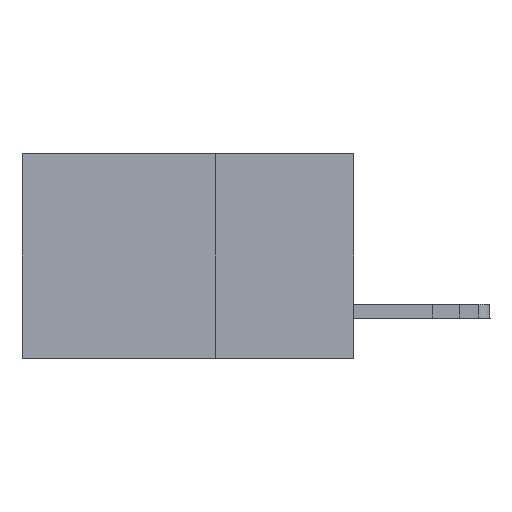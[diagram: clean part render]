
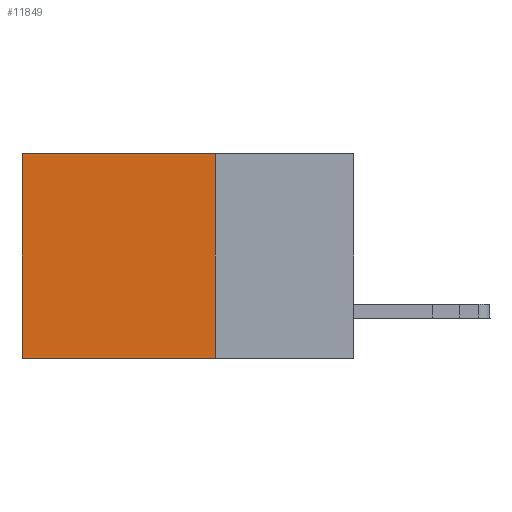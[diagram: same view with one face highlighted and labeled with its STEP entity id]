
A CAD part, left-side view. The second image highlights one B-rep face of the part: STEP entity #11849.
In plain terms, the highlighted planar face has unit normal (-1, 0, 0).
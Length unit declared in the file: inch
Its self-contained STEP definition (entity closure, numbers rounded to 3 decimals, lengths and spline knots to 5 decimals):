
#397 = DIRECTION ( 'NONE',  ( 0., 1., 0. ) ) ;
#1857 = CARTESIAN_POINT ( 'NONE',  ( 0.2875, 0.6, 0. ) ) ;
#2567 = VECTOR ( 'NONE', #23608, 39.37008 ) ;
#2897 = ORIENTED_EDGE ( 'NONE', *, *, #4030, .F. ) ;
#2952 = CARTESIAN_POINT ( 'NONE',  ( 0.2875, 0.25, 0. ) ) ;
#3026 = LINE ( 'NONE', #13489, #25670 ) ;
#3095 = ORIENTED_EDGE ( 'NONE', *, *, #11351, .T. ) ;
#3740 = VECTOR ( 'NONE', #397, 39.37008 ) ;
#4030 = EDGE_CURVE ( 'NONE', #10977, #20975, #3026, .T. ) ;
#5952 = VERTEX_POINT ( 'NONE', #2952 ) ;
#7763 = EDGE_CURVE ( 'NONE', #5952, #10977, #14908, .T. ) ;
#9144 = EDGE_CURVE ( 'NONE', #24712, #20975, #12087, .T. ) ;
#10121 = CARTESIAN_POINT ( 'NONE',  ( 0.2875, 0.25, -0.37 ) ) ;
#10652 = DIRECTION ( 'NONE',  ( 1., 0., 0. ) ) ;
#10977 = VERTEX_POINT ( 'NONE', #10121 ) ;
#11351 = EDGE_CURVE ( 'NONE', #5952, #24712, #21190, .T. ) ;
#11849 = ADVANCED_FACE ( 'NONE', ( #12816 ), #26188, .F. ) ;
#12087 = LINE ( 'NONE', #15108, #17179 ) ;
#12816 = FACE_OUTER_BOUND ( 'NONE', #22720, .T. ) ;
#13489 = CARTESIAN_POINT ( 'NONE',  ( 0.2875, 0.25, -0.37 ) ) ;
#14557 = ORIENTED_EDGE ( 'NONE', *, *, #7763, .F. ) ;
#14908 = LINE ( 'NONE', #21387, #2567 ) ;
#15108 = CARTESIAN_POINT ( 'NONE',  ( 0.2875, 0.6, 0. ) ) ;
#17179 = VECTOR ( 'NONE', #17284, 39.37008 ) ;
#17284 = DIRECTION ( 'NONE',  ( 0., 0., -1. ) ) ;
#17630 = ORIENTED_EDGE ( 'NONE', *, *, #9144, .T. ) ;
#20975 = VERTEX_POINT ( 'NONE', #26289 ) ;
#21190 = LINE ( 'NONE', #26684, #3740 ) ;
#21387 = CARTESIAN_POINT ( 'NONE',  ( 0.2875, 0.25, 0. ) ) ;
#22720 = EDGE_LOOP ( 'NONE', ( #17630, #2897, #14557, #3095 ) ) ;
#23608 = DIRECTION ( 'NONE',  ( 0., 0., -1. ) ) ;
#23948 = CARTESIAN_POINT ( 'NONE',  ( 0.2875, 0.25, 0. ) ) ;
#24712 = VERTEX_POINT ( 'NONE', #1857 ) ;
#25670 = VECTOR ( 'NONE', #26637, 39.37008 ) ;
#26188 = PLANE ( 'NONE',  #26867 ) ;
#26289 = CARTESIAN_POINT ( 'NONE',  ( 0.2875, 0.6, -0.37 ) ) ;
#26637 = DIRECTION ( 'NONE',  ( 0., 1., 0. ) ) ;
#26684 = CARTESIAN_POINT ( 'NONE',  ( 0.2875, 0.25, 0. ) ) ;
#26867 = AXIS2_PLACEMENT_3D ( 'NONE', #23948, #10652, #28397 ) ;
#28397 = DIRECTION ( 'NONE',  ( 0., 0., -1. ) ) ;
